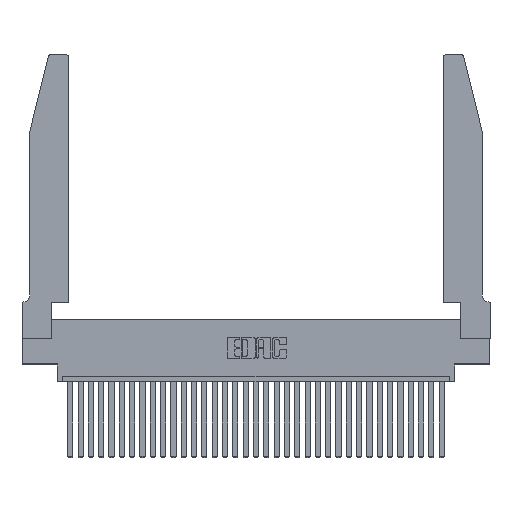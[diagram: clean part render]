
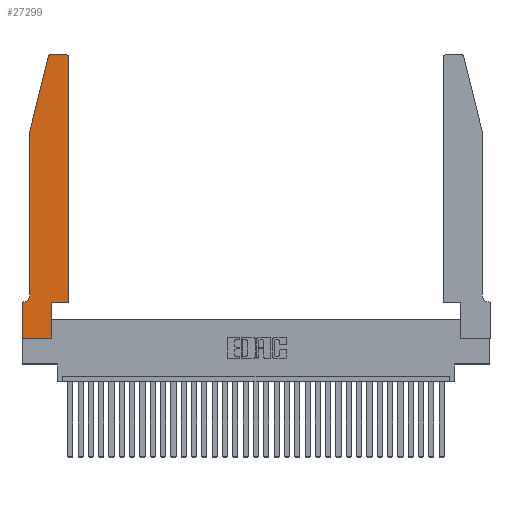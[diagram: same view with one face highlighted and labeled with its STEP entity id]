
A CAD part, top view. The second image highlights one B-rep face of the part: STEP entity #27299.
In plain terms, the highlighted planar face has unit normal (0, 0, 1).
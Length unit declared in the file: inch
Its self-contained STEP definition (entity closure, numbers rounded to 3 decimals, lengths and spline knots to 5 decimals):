
#5 = ORIENTED_EDGE ( 'NONE', *, *, #19437, .T. ) ;
#459 = VERTEX_POINT ( 'NONE', #2992 ) ;
#610 = VERTEX_POINT ( 'NONE', #19176 ) ;
#629 = DIRECTION ( 'NONE',  ( -1., 0., 0. ) ) ;
#1255 = PLANE ( 'NONE',  #7958 ) ;
#1472 = LINE ( 'NONE', #9108, #24713 ) ;
#1490 = EDGE_CURVE ( 'NONE', #9550, #20173, #11868, .T. ) ;
#1641 = VECTOR ( 'NONE', #16202, 39.37008 ) ;
#2165 = DIRECTION ( 'NONE',  ( -0.239, -0.971, 0. ) ) ;
#2463 = LINE ( 'NONE', #10263, #3256 ) ;
#2992 = CARTESIAN_POINT ( 'NONE',  ( 0.4205, 2.75, 0.37 ) ) ;
#3028 = ORIENTED_EDGE ( 'NONE', *, *, #8100, .T. ) ;
#3256 = VECTOR ( 'NONE', #28130, 39.37008 ) ;
#3317 = FACE_OUTER_BOUND ( 'NONE', #29718, .T. ) ;
#3618 = CARTESIAN_POINT ( 'NONE',  ( 0.284, 2.75, 0.37 ) ) ;
#3723 = CARTESIAN_POINT ( 'NONE',  ( 0.2865, 0.35, 0.37 ) ) ;
#3824 = EDGE_CURVE ( 'NONE', #22783, #24745, #8333, .T. ) ;
#4325 = CARTESIAN_POINT ( 'NONE',  ( 0.4505, 0.35, 0.37 ) ) ;
#5809 = CARTESIAN_POINT ( 'NONE',  ( 0.4505, 0.35, 0.37 ) ) ;
#6015 = CIRCLE ( 'NONE', #30250, 0.07 ) ;
#6245 = CIRCLE ( 'NONE', #28364, 0.03 ) ;
#6350 = VERTEX_POINT ( 'NONE', #9885 ) ;
#6412 = CARTESIAN_POINT ( 'NONE',  ( 0., 0.35, 0.37 ) ) ;
#6567 = LINE ( 'NONE', #32702, #33032 ) ;
#6717 = VERTEX_POINT ( 'NONE', #11340 ) ;
#7148 = DIRECTION ( 'NONE',  ( 1., 0., 0. ) ) ;
#7334 = LINE ( 'NONE', #28699, #1641 ) ;
#7396 = CARTESIAN_POINT ( 'NONE',  ( 0.0755, 0.42, 0.37 ) ) ;
#7509 = CARTESIAN_POINT ( 'NONE',  ( 0.0755, 0.35, 0.37 ) ) ;
#7786 = DIRECTION ( 'NONE',  ( 1., 0., 0. ) ) ;
#7958 = AXIS2_PLACEMENT_3D ( 'NONE', #6412, #26988, #14312 ) ;
#8043 = DIRECTION ( 'NONE',  ( 0., 1., 0. ) ) ;
#8100 = EDGE_CURVE ( 'NONE', #20173, #26833, #19363, .T. ) ;
#8333 = LINE ( 'NONE', #7509, #16430 ) ;
#9108 = CARTESIAN_POINT ( 'NONE',  ( 0., 0., 0.37 ) ) ;
#9550 = VERTEX_POINT ( 'NONE', #3618 ) ;
#9797 = EDGE_CURVE ( 'NONE', #459, #9550, #30245, .T. ) ;
#9885 = CARTESIAN_POINT ( 'NONE',  ( 0.2865, 0., 0.37 ) ) ;
#9917 = DIRECTION ( 'NONE',  ( 0., 0., 1. ) ) ;
#10263 = CARTESIAN_POINT ( 'NONE',  ( 0.0755, 2., 0.37 ) ) ;
#10563 = EDGE_CURVE ( 'NONE', #6350, #6717, #13014, .T. ) ;
#11340 = CARTESIAN_POINT ( 'NONE',  ( 0.2865, 0.35, 0.37 ) ) ;
#11868 = CIRCLE ( 'NONE', #26032, 0.03 ) ;
#13014 = LINE ( 'NONE', #3723, #24976 ) ;
#13044 = CARTESIAN_POINT ( 'NONE',  ( 0., 0., 0.37 ) ) ;
#13787 = ORIENTED_EDGE ( 'NONE', *, *, #18424, .T. ) ;
#14062 = ORIENTED_EDGE ( 'NONE', *, *, #3824, .T. ) ;
#14261 = VERTEX_POINT ( 'NONE', #4325 ) ;
#14312 = DIRECTION ( 'NONE',  ( 1., 0., 0. ) ) ;
#14803 = DIRECTION ( 'NONE',  ( 0., 0., 1. ) ) ;
#16167 = EDGE_CURVE ( 'NONE', #6717, #14261, #7334, .T. ) ;
#16202 = DIRECTION ( 'NONE',  ( 1., 0., 0. ) ) ;
#16430 = VECTOR ( 'NONE', #17424, 39.37008 ) ;
#16768 = CARTESIAN_POINT ( 'NONE',  ( 0.0055, 0.35, 0.37 ) ) ;
#16782 = VERTEX_POINT ( 'NONE', #7396 ) ;
#17424 = DIRECTION ( 'NONE',  ( -1., 0., 0. ) ) ;
#17514 = ORIENTED_EDGE ( 'NONE', *, *, #1490, .T. ) ;
#17596 = VERTEX_POINT ( 'NONE', #13044 ) ;
#18424 = EDGE_CURVE ( 'NONE', #17596, #6350, #6567, .T. ) ;
#19164 = ORIENTED_EDGE ( 'NONE', *, *, #28339, .T. ) ;
#19176 = CARTESIAN_POINT ( 'NONE',  ( 0.4505, 2.72, 0.37 ) ) ;
#19363 = LINE ( 'NONE', #30397, #24518 ) ;
#19437 = EDGE_CURVE ( 'NONE', #16782, #22783, #6015, .T. ) ;
#19546 = CARTESIAN_POINT ( 'NONE',  ( 0.4205, 2.72, 0.37 ) ) ;
#19891 = CARTESIAN_POINT ( 'NONE',  ( 0.2605, 2.75, 0.37 ) ) ;
#19905 = CARTESIAN_POINT ( 'NONE',  ( 0.0755, 2., 0.37 ) ) ;
#20173 = VERTEX_POINT ( 'NONE', #29071 ) ;
#21896 = CARTESIAN_POINT ( 'NONE',  ( 0., 0.35, 0.37 ) ) ;
#21913 = EDGE_CURVE ( 'NONE', #610, #459, #6245, .T. ) ;
#21987 = ORIENTED_EDGE ( 'NONE', *, *, #9797, .T. ) ;
#22045 = ORIENTED_EDGE ( 'NONE', *, *, #10563, .T. ) ;
#22783 = VERTEX_POINT ( 'NONE', #16768 ) ;
#22838 = VECTOR ( 'NONE', #8043, 39.37008 ) ;
#22866 = DIRECTION ( 'NONE',  ( 1., 0., 0. ) ) ;
#23011 = VECTOR ( 'NONE', #27787, 39.37008 ) ;
#23385 = ORIENTED_EDGE ( 'NONE', *, *, #16167, .T. ) ;
#24145 = CARTESIAN_POINT ( 'NONE',  ( 0.0055, 0.42, 0.37 ) ) ;
#24518 = VECTOR ( 'NONE', #2165, 39.37008 ) ;
#24713 = VECTOR ( 'NONE', #32309, 39.37008 ) ;
#24745 = VERTEX_POINT ( 'NONE', #21896 ) ;
#24868 = LINE ( 'NONE', #5809, #22838 ) ;
#24976 = VECTOR ( 'NONE', #31663, 39.37008 ) ;
#25225 = ORIENTED_EDGE ( 'NONE', *, *, #21913, .T. ) ;
#26032 = AXIS2_PLACEMENT_3D ( 'NONE', #27684, #9917, #22866 ) ;
#26833 = VERTEX_POINT ( 'NONE', #19905 ) ;
#26988 = DIRECTION ( 'NONE',  ( 0., 0., 1. ) ) ;
#27299 = ADVANCED_FACE ( 'NONE', ( #3317 ), #1255, .T. ) ;
#27684 = CARTESIAN_POINT ( 'NONE',  ( 0.284, 2.72, 0.37 ) ) ;
#27787 = DIRECTION ( 'NONE',  ( -1., 0., 0. ) ) ;
#28130 = DIRECTION ( 'NONE',  ( 0., -1., 0. ) ) ;
#28339 = EDGE_CURVE ( 'NONE', #26833, #16782, #2463, .T. ) ;
#28364 = AXIS2_PLACEMENT_3D ( 'NONE', #19546, #14803, #7786 ) ;
#28699 = CARTESIAN_POINT ( 'NONE',  ( 0.4505, 0.35, 0.37 ) ) ;
#28958 = DIRECTION ( 'NONE',  ( 0., 0., -1. ) ) ;
#29071 = CARTESIAN_POINT ( 'NONE',  ( 0.25487, 2.72718, 0.37 ) ) ;
#29124 = EDGE_CURVE ( 'NONE', #14261, #610, #24868, .T. ) ;
#29370 = ORIENTED_EDGE ( 'NONE', *, *, #29124, .T. ) ;
#29429 = ORIENTED_EDGE ( 'NONE', *, *, #30893, .T. ) ;
#29718 = EDGE_LOOP ( 'NONE', ( #21987, #17514, #3028, #19164, #5, #14062, #29429, #13787, #22045, #23385, #29370, #25225 ) ) ;
#30245 = LINE ( 'NONE', #19891, #23011 ) ;
#30250 = AXIS2_PLACEMENT_3D ( 'NONE', #24145, #28958, #629 ) ;
#30397 = CARTESIAN_POINT ( 'NONE',  ( 0.0755, 2., 0.37 ) ) ;
#30893 = EDGE_CURVE ( 'NONE', #24745, #17596, #1472, .T. ) ;
#31663 = DIRECTION ( 'NONE',  ( 0., 1., 0. ) ) ;
#32309 = DIRECTION ( 'NONE',  ( 0., -1., 0. ) ) ;
#32702 = CARTESIAN_POINT ( 'NONE',  ( 0., 0., 0.37 ) ) ;
#33032 = VECTOR ( 'NONE', #7148, 39.37008 ) ;
